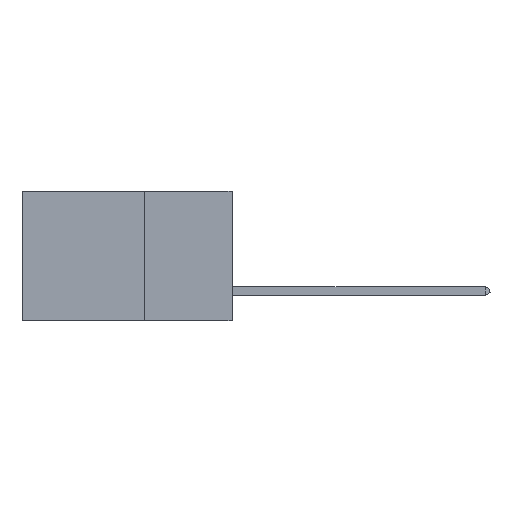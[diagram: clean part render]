
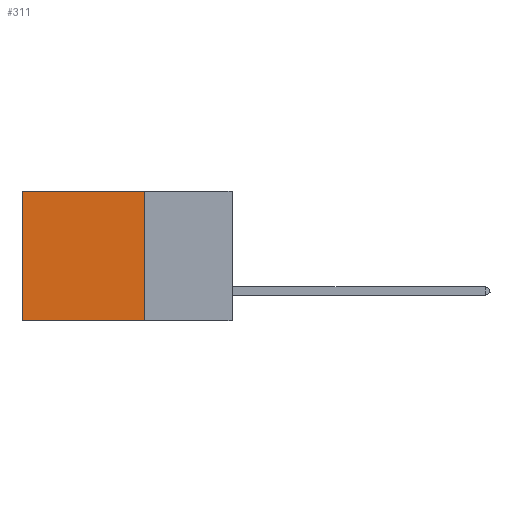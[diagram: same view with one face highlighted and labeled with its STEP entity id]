
A CAD part, left-side view. The second image highlights one B-rep face of the part: STEP entity #311.
In plain terms, the highlighted planar face has unit normal (-1, 0, 0).
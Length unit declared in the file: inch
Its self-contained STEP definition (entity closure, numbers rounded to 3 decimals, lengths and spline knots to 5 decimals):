
#55 = AXIS2_PLACEMENT_3D ( 'NONE', #6086, #2231, #12826 ) ;
#172 = VECTOR ( 'NONE', #1551, 39.37008 ) ;
#311 = ADVANCED_FACE ( 'NONE', ( #3810 ), #8853, .F. ) ;
#1551 = DIRECTION ( 'NONE',  ( 0., 1., 0. ) ) ;
#2231 = DIRECTION ( 'NONE',  ( 1., 0., 0. ) ) ;
#2494 = CARTESIAN_POINT ( 'NONE',  ( 0.2875, 0.25, 0. ) ) ;
#2568 = EDGE_CURVE ( 'NONE', #14193, #8661, #7924, .T. ) ;
#3474 = VERTEX_POINT ( 'NONE', #10856 ) ;
#3810 = FACE_OUTER_BOUND ( 'NONE', #4226, .T. ) ;
#4175 = CARTESIAN_POINT ( 'NONE',  ( 0.2875, 0.25, -0.37 ) ) ;
#4226 = EDGE_LOOP ( 'NONE', ( #4525, #11153, #16502, #14351 ) ) ;
#4525 = ORIENTED_EDGE ( 'NONE', *, *, #16137, .T. ) ;
#5257 = DIRECTION ( 'NONE',  ( 0., 0., -1. ) ) ;
#5436 = VECTOR ( 'NONE', #6411, 39.37008 ) ;
#5695 = CARTESIAN_POINT ( 'NONE',  ( 0.2875, 0.25, 0. ) ) ;
#5854 = VECTOR ( 'NONE', #12383, 39.37008 ) ;
#6086 = CARTESIAN_POINT ( 'NONE',  ( 0.2875, 0.25, 0. ) ) ;
#6411 = DIRECTION ( 'NONE',  ( 0., 0., -1. ) ) ;
#6481 = LINE ( 'NONE', #5695, #5854 ) ;
#7924 = LINE ( 'NONE', #2494, #5436 ) ;
#8661 = VERTEX_POINT ( 'NONE', #16094 ) ;
#8853 = PLANE ( 'NONE',  #55 ) ;
#9290 = EDGE_CURVE ( 'NONE', #14193, #3474, #6481, .T. ) ;
#9471 = CARTESIAN_POINT ( 'NONE',  ( 0.2875, 0.6, -0.37 ) ) ;
#10856 = CARTESIAN_POINT ( 'NONE',  ( 0.2875, 0.6, 0. ) ) ;
#11153 = ORIENTED_EDGE ( 'NONE', *, *, #11429, .F. ) ;
#11429 = EDGE_CURVE ( 'NONE', #8661, #13236, #14255, .T. ) ;
#12383 = DIRECTION ( 'NONE',  ( 0., 1., 0. ) ) ;
#12826 = DIRECTION ( 'NONE',  ( 0., 0., -1. ) ) ;
#12903 = CARTESIAN_POINT ( 'NONE',  ( 0.2875, 0.25, 0. ) ) ;
#13122 = CARTESIAN_POINT ( 'NONE',  ( 0.2875, 0.6, 0. ) ) ;
#13236 = VERTEX_POINT ( 'NONE', #9471 ) ;
#13396 = LINE ( 'NONE', #13122, #14662 ) ;
#14193 = VERTEX_POINT ( 'NONE', #12903 ) ;
#14255 = LINE ( 'NONE', #4175, #172 ) ;
#14351 = ORIENTED_EDGE ( 'NONE', *, *, #9290, .T. ) ;
#14662 = VECTOR ( 'NONE', #5257, 39.37008 ) ;
#16094 = CARTESIAN_POINT ( 'NONE',  ( 0.2875, 0.25, -0.37 ) ) ;
#16137 = EDGE_CURVE ( 'NONE', #3474, #13236, #13396, .T. ) ;
#16502 = ORIENTED_EDGE ( 'NONE', *, *, #2568, .F. ) ;
